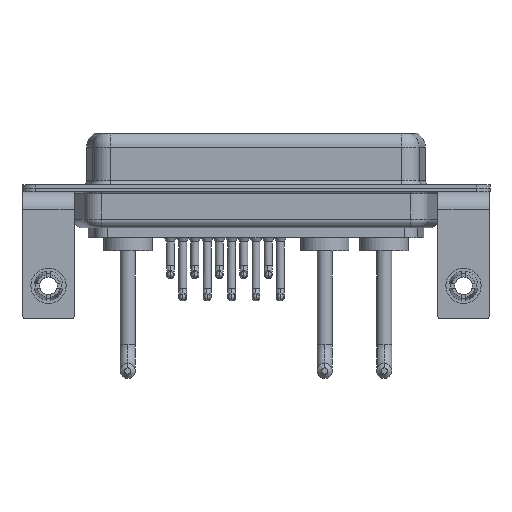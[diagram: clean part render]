
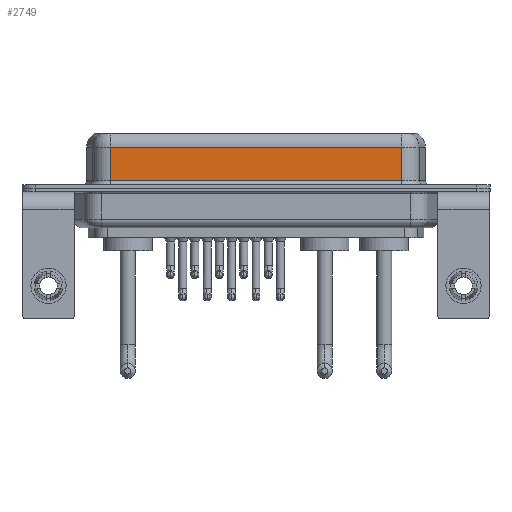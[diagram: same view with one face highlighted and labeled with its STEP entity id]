
A CAD part, front view. The second image highlights one B-rep face of the part: STEP entity #2749.
In plain terms, the highlighted planar face has unit normal (0, -1, 0).
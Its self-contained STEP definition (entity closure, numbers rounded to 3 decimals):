
#33 = CARTESIAN_POINT ( 'NONE',  ( 7.013, -3.95, 4.65 ) ) ;
#1041 = CARTESIAN_POINT ( 'NONE',  ( 40.037, -3.95, 6.4 ) ) ;
#1477 = EDGE_CURVE ( 'NONE', #20709, #12622, #18584, .T. ) ;
#2749 = ADVANCED_FACE ( 'NONE', ( #12552 ), #15913, .F. ) ;
#3422 = EDGE_CURVE ( 'NONE', #4509, #14395, #7816, .T. ) ;
#3424 = LINE ( 'NONE', #14695, #13965 ) ;
#4356 = CARTESIAN_POINT ( 'NONE',  ( 40.037, -3.95, 0.9 ) ) ;
#4509 = VERTEX_POINT ( 'NONE', #10119 ) ;
#4755 = VECTOR ( 'NONE', #16191, 1000. ) ;
#5260 = CARTESIAN_POINT ( 'NONE',  ( 40.037, -3.95, 4.65 ) ) ;
#6403 = ORIENTED_EDGE ( 'NONE', *, *, #3422, .T. ) ;
#6675 = DIRECTION ( 'NONE',  ( -1., 0., 0. ) ) ;
#7327 = CARTESIAN_POINT ( 'NONE',  ( 40.037, -3.95, 4.65 ) ) ;
#7816 = LINE ( 'NONE', #4356, #9967 ) ;
#9596 = CARTESIAN_POINT ( 'NONE',  ( 40.037, -3.95, 6.4 ) ) ;
#9745 = ORIENTED_EDGE ( 'NONE', *, *, #15508, .T. ) ;
#9967 = VECTOR ( 'NONE', #11393, 1000. ) ;
#10119 = CARTESIAN_POINT ( 'NONE',  ( 7.013, -3.95, 0.9 ) ) ;
#10632 = EDGE_CURVE ( 'NONE', #20709, #14395, #14461, .T. ) ;
#11242 = ORIENTED_EDGE ( 'NONE', *, *, #1477, .T. ) ;
#11393 = DIRECTION ( 'NONE',  ( 1., 0., 0. ) ) ;
#12552 = FACE_OUTER_BOUND ( 'NONE', #16563, .T. ) ;
#12622 = VERTEX_POINT ( 'NONE', #33 ) ;
#13965 = VECTOR ( 'NONE', #14803, 1000. ) ;
#14395 = VERTEX_POINT ( 'NONE', #17846 ) ;
#14461 = LINE ( 'NONE', #9596, #4755 ) ;
#14695 = CARTESIAN_POINT ( 'NONE',  ( 7.013, -3.95, 6.4 ) ) ;
#14704 = ORIENTED_EDGE ( 'NONE', *, *, #10632, .F. ) ;
#14803 = DIRECTION ( 'NONE',  ( 0., 0., -1. ) ) ;
#15508 = EDGE_CURVE ( 'NONE', #12622, #4509, #3424, .T. ) ;
#15913 = PLANE ( 'NONE',  #20650 ) ;
#16191 = DIRECTION ( 'NONE',  ( 0., 0., -1. ) ) ;
#16563 = EDGE_LOOP ( 'NONE', ( #14704, #11242, #9745, #6403 ) ) ;
#17846 = CARTESIAN_POINT ( 'NONE',  ( 40.037, -3.95, 0.9 ) ) ;
#18584 = LINE ( 'NONE', #5260, #19215 ) ;
#19156 = DIRECTION ( 'NONE',  ( 0., 0., 1. ) ) ;
#19215 = VECTOR ( 'NONE', #6675, 1000. ) ;
#19379 = DIRECTION ( 'NONE',  ( 0., 1., 0. ) ) ;
#20650 = AXIS2_PLACEMENT_3D ( 'NONE', #1041, #19379, #19156 ) ;
#20709 = VERTEX_POINT ( 'NONE', #7327 ) ;
